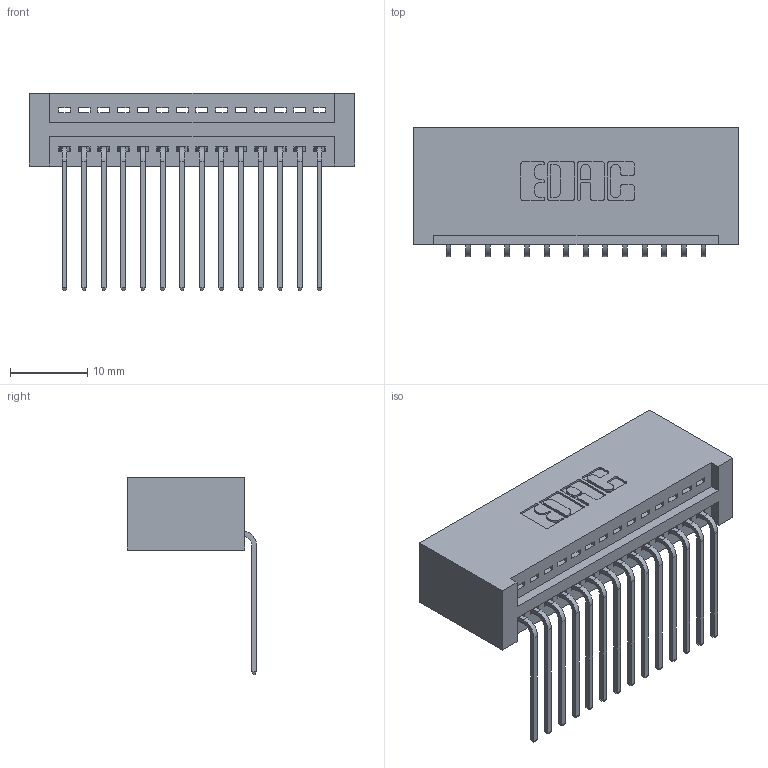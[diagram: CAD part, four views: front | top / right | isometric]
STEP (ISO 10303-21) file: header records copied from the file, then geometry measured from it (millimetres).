
FILE_DESCRIPTION (( 'STEP AP203' ), '1' );
FILE_NAME ('395-014-559-101.STEP', '2019-10-16T05:24:52', ( '' ), ( '' ), 'SwSTEP 2.0', 'SolidWorks 2016', '' );
FILE_SCHEMA (( 'CONFIG_CONTROL_DESIGN' ));
Length unit declared in the file: inch
Products named in the file (3): 395-014-559-101; 345-292-001_558 559 Tail - 1; 345 Part_No Mounting Lugs
Assembly tree (15 placements, depth 2):
  395-014-559-101
    345 Part_No Mounting Lugs
    345-292-001_558 559 Tail - 1  x14
Bounding box: 42.16 x 16.75 x 25.53 mm (x, y, z)
Volume: 4406.4 mm3; surface area: 5939.4 mm2
Topology: 15 solids, 15 shells, 958 faces, 2865 edges, 1890 vertices
Faces by surface type: plane 664, cylinder 294
Entity records: 14113 total; most frequent: CARTESIAN_POINT 2454, ORIENTED_EDGE 2402, DIRECTION 2177, EDGE_CURVE 1201, LINE 1021, VECTOR 1021, VERTEX_POINT 798, AXIS2_PLACEMENT_3D 578
